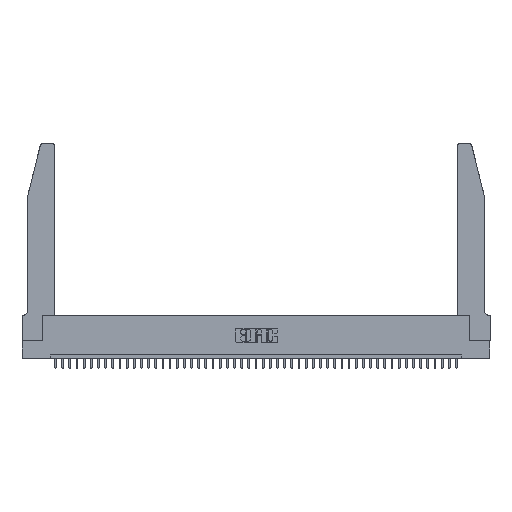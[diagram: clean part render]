
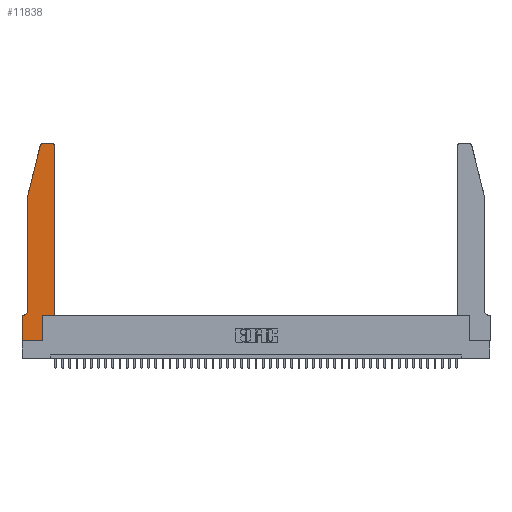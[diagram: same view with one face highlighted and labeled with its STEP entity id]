
A CAD part, top view. The second image highlights one B-rep face of the part: STEP entity #11838.
In plain terms, the highlighted planar face has unit normal (0, 0, 1).
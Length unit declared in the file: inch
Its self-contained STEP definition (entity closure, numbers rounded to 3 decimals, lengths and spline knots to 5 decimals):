
#552 = LINE ( 'NONE', #32044, #19992 ) ;
#892 = DIRECTION ( 'NONE',  ( 0., 0., -1. ) ) ;
#932 = VECTOR ( 'NONE', #41573, 39.37008 ) ;
#980 = VECTOR ( 'NONE', #22114, 39.37008 ) ;
#1197 = DIRECTION ( 'NONE',  ( 0., 0., 1. ) ) ;
#1498 = DIRECTION ( 'NONE',  ( 1., 0., 0. ) ) ;
#1761 = CARTESIAN_POINT ( 'NONE',  ( 0.2605, 2.75, 0.37 ) ) ;
#1874 = CARTESIAN_POINT ( 'NONE',  ( 0.4505, 0.35, 0.37 ) ) ;
#2167 = DIRECTION ( 'NONE',  ( 1., 0., 0. ) ) ;
#2201 = CARTESIAN_POINT ( 'NONE',  ( 0.4205, 2.75, 0.37 ) ) ;
#2349 = CARTESIAN_POINT ( 'NONE',  ( 0.0755, 2., 0.37 ) ) ;
#2863 = LINE ( 'NONE', #1761, #23294 ) ;
#4110 = EDGE_CURVE ( 'NONE', #42356, #4744, #16498, .T. ) ;
#4744 = VERTEX_POINT ( 'NONE', #26711 ) ;
#5651 = ORIENTED_EDGE ( 'NONE', *, *, #20258, .T. ) ;
#5831 = AXIS2_PLACEMENT_3D ( 'NONE', #22372, #1197, #25884 ) ;
#6102 = VECTOR ( 'NONE', #16599, 39.37008 ) ;
#6525 = LINE ( 'NONE', #6779, #932 ) ;
#6736 = ORIENTED_EDGE ( 'NONE', *, *, #31641, .T. ) ;
#6779 = CARTESIAN_POINT ( 'NONE',  ( 0., 0., 0.37 ) ) ;
#7248 = VERTEX_POINT ( 'NONE', #37712 ) ;
#8067 = EDGE_CURVE ( 'NONE', #4744, #24327, #42075, .T. ) ;
#9018 = ORIENTED_EDGE ( 'NONE', *, *, #25697, .T. ) ;
#9500 = CARTESIAN_POINT ( 'NONE',  ( 0.0755, 0.35, 0.37 ) ) ;
#9523 = EDGE_CURVE ( 'NONE', #9878, #38537, #38968, .T. ) ;
#9651 = CARTESIAN_POINT ( 'NONE',  ( 0.4205, 2.72, 0.37 ) ) ;
#9878 = VERTEX_POINT ( 'NONE', #21831 ) ;
#10706 = ORIENTED_EDGE ( 'NONE', *, *, #34651, .T. ) ;
#11838 = ADVANCED_FACE ( 'NONE', ( #16740 ), #15222, .T. ) ;
#12049 = EDGE_CURVE ( 'NONE', #24327, #28958, #40959, .T. ) ;
#12641 = LINE ( 'NONE', #39007, #980 ) ;
#13627 = EDGE_CURVE ( 'NONE', #19580, #9878, #552, .T. ) ;
#14632 = AXIS2_PLACEMENT_3D ( 'NONE', #33749, #19806, #2167 ) ;
#15222 = PLANE ( 'NONE',  #5831 ) ;
#15948 = ORIENTED_EDGE ( 'NONE', *, *, #8067, .T. ) ;
#16498 = LINE ( 'NONE', #21896, #18680 ) ;
#16599 = DIRECTION ( 'NONE',  ( -1., 0., 0. ) ) ;
#16740 = FACE_OUTER_BOUND ( 'NONE', #35000, .T. ) ;
#17195 = DIRECTION ( 'NONE',  ( 1., 0., 0. ) ) ;
#17213 = VERTEX_POINT ( 'NONE', #32575 ) ;
#17332 = CARTESIAN_POINT ( 'NONE',  ( 0.2865, 0.35, 0.37 ) ) ;
#17404 = ORIENTED_EDGE ( 'NONE', *, *, #31321, .T. ) ;
#18680 = VECTOR ( 'NONE', #1498, 39.37008 ) ;
#19040 = DIRECTION ( 'NONE',  ( 0., 1., 0. ) ) ;
#19414 = ORIENTED_EDGE ( 'NONE', *, *, #13627, .T. ) ;
#19580 = VERTEX_POINT ( 'NONE', #42003 ) ;
#19592 = EDGE_CURVE ( 'NONE', #17213, #42356, #12641, .T. ) ;
#19670 = DIRECTION ( 'NONE',  ( 0., -1., 0. ) ) ;
#19806 = DIRECTION ( 'NONE',  ( 0., 0., 1. ) ) ;
#19992 = VECTOR ( 'NONE', #25090, 39.37008 ) ;
#20039 = AXIS2_PLACEMENT_3D ( 'NONE', #9651, #30302, #34118 ) ;
#20258 = EDGE_CURVE ( 'NONE', #21272, #24382, #6525, .T. ) ;
#20259 = CARTESIAN_POINT ( 'NONE',  ( 0., 0.35, 0.37 ) ) ;
#21272 = VERTEX_POINT ( 'NONE', #20259 ) ;
#21673 = VECTOR ( 'NONE', #19040, 39.37008 ) ;
#21831 = CARTESIAN_POINT ( 'NONE',  ( 0.0755, 2., 0.37 ) ) ;
#21896 = CARTESIAN_POINT ( 'NONE',  ( 0.4505, 0.35, 0.37 ) ) ;
#22114 = DIRECTION ( 'NONE',  ( 0., 1., 0. ) ) ;
#22190 = AXIS2_PLACEMENT_3D ( 'NONE', #22681, #892, #43250 ) ;
#22371 = LINE ( 'NONE', #31258, #38847 ) ;
#22372 = CARTESIAN_POINT ( 'NONE',  ( 0., 0.35, 0.37 ) ) ;
#22588 = EDGE_CURVE ( 'NONE', #7248, #19580, #28457, .T. ) ;
#22681 = CARTESIAN_POINT ( 'NONE',  ( 0.0055, 0.42, 0.37 ) ) ;
#23294 = VECTOR ( 'NONE', #33216, 39.37008 ) ;
#24327 = VERTEX_POINT ( 'NONE', #36888 ) ;
#24382 = VERTEX_POINT ( 'NONE', #33267 ) ;
#24958 = CIRCLE ( 'NONE', #22190, 0.07 ) ;
#25090 = DIRECTION ( 'NONE',  ( -0.239, -0.971, 0. ) ) ;
#25697 = EDGE_CURVE ( 'NONE', #33751, #21272, #31499, .T. ) ;
#25884 = DIRECTION ( 'NONE',  ( 1., 0., 0. ) ) ;
#26178 = ORIENTED_EDGE ( 'NONE', *, *, #22588, .T. ) ;
#26711 = CARTESIAN_POINT ( 'NONE',  ( 0.4505, 0.35, 0.37 ) ) ;
#28163 = ORIENTED_EDGE ( 'NONE', *, *, #9523, .T. ) ;
#28457 = CIRCLE ( 'NONE', #14632, 0.03 ) ;
#28958 = VERTEX_POINT ( 'NONE', #2201 ) ;
#29661 = VECTOR ( 'NONE', #19670, 39.37008 ) ;
#29936 = ORIENTED_EDGE ( 'NONE', *, *, #19592, .T. ) ;
#30302 = DIRECTION ( 'NONE',  ( 0., 0., 1. ) ) ;
#31258 = CARTESIAN_POINT ( 'NONE',  ( 0., 0., 0.37 ) ) ;
#31321 = EDGE_CURVE ( 'NONE', #28958, #7248, #2863, .T. ) ;
#31460 = CARTESIAN_POINT ( 'NONE',  ( 0.0755, 0.42, 0.37 ) ) ;
#31499 = LINE ( 'NONE', #9500, #6102 ) ;
#31641 = EDGE_CURVE ( 'NONE', #24382, #17213, #22371, .T. ) ;
#32044 = CARTESIAN_POINT ( 'NONE',  ( 0.0755, 2., 0.37 ) ) ;
#32575 = CARTESIAN_POINT ( 'NONE',  ( 0.2865, 0., 0.37 ) ) ;
#33216 = DIRECTION ( 'NONE',  ( -1., 0., 0. ) ) ;
#33267 = CARTESIAN_POINT ( 'NONE',  ( 0., 0., 0.37 ) ) ;
#33749 = CARTESIAN_POINT ( 'NONE',  ( 0.284, 2.72, 0.37 ) ) ;
#33751 = VERTEX_POINT ( 'NONE', #41869 ) ;
#34118 = DIRECTION ( 'NONE',  ( 1., 0., 0. ) ) ;
#34651 = EDGE_CURVE ( 'NONE', #38537, #33751, #24958, .T. ) ;
#35000 = EDGE_LOOP ( 'NONE', ( #17404, #26178, #19414, #28163, #10706, #9018, #5651, #6736, #29936, #38695, #15948, #36170 ) ) ;
#36170 = ORIENTED_EDGE ( 'NONE', *, *, #12049, .T. ) ;
#36888 = CARTESIAN_POINT ( 'NONE',  ( 0.4505, 2.72, 0.37 ) ) ;
#37712 = CARTESIAN_POINT ( 'NONE',  ( 0.284, 2.75, 0.37 ) ) ;
#38537 = VERTEX_POINT ( 'NONE', #31460 ) ;
#38695 = ORIENTED_EDGE ( 'NONE', *, *, #4110, .T. ) ;
#38847 = VECTOR ( 'NONE', #17195, 39.37008 ) ;
#38968 = LINE ( 'NONE', #2349, #29661 ) ;
#39007 = CARTESIAN_POINT ( 'NONE',  ( 0.2865, 0.35, 0.37 ) ) ;
#40959 = CIRCLE ( 'NONE', #20039, 0.03 ) ;
#41573 = DIRECTION ( 'NONE',  ( 0., -1., 0. ) ) ;
#41869 = CARTESIAN_POINT ( 'NONE',  ( 0.0055, 0.35, 0.37 ) ) ;
#42003 = CARTESIAN_POINT ( 'NONE',  ( 0.25487, 2.72718, 0.37 ) ) ;
#42075 = LINE ( 'NONE', #1874, #21673 ) ;
#42356 = VERTEX_POINT ( 'NONE', #17332 ) ;
#43250 = DIRECTION ( 'NONE',  ( -1., 0., 0. ) ) ;
